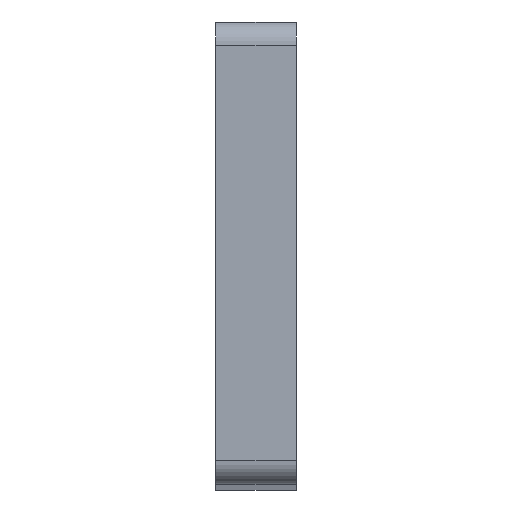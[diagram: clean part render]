
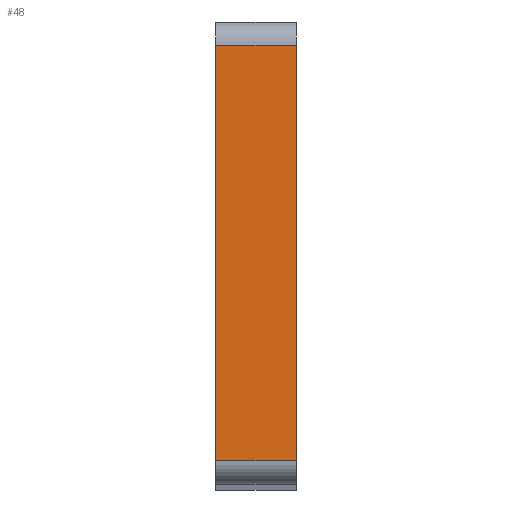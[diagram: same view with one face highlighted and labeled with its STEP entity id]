
A CAD part, top view. The second image highlights one B-rep face of the part: STEP entity #48.
In plain terms, the highlighted planar face has unit normal (0, 0, 1).
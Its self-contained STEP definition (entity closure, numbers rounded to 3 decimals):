
#1 = VERTEX_POINT ( 'NONE', #144 ) ;
#2 = VERTEX_POINT ( 'NONE', #148 ) ;
#8 = VERTEX_POINT ( 'NONE', #146 ) ;
#9 = VERTEX_POINT ( 'NONE', #147 ) ;
#19 = ORIENTED_EDGE ( 'NONE', *, *, #415, .T. ) ;
#26 = ORIENTED_EDGE ( 'NONE', *, *, #418, .T. ) ;
#28 = EDGE_LOOP ( 'NONE', ( #341, #26, #19, #34 ) ) ;
#34 = ORIENTED_EDGE ( 'NONE', *, *, #409, .T. ) ;
#48 = ADVANCED_FACE ( 'NONE', ( #291 ), #127, .F. ) ;
#124 = DIRECTION ( 'NONE',  ( -1., 0., 0. ) ) ;
#125 = DIRECTION ( 'NONE',  ( 0., 0., -1. ) ) ;
#127 = PLANE ( 'NONE',  #198 ) ;
#135 = CARTESIAN_POINT ( 'NONE',  ( 0.7, 0., 34. ) ) ;
#144 = CARTESIAN_POINT ( 'NONE',  ( 0., 3.8, 34. ) ) ;
#146 = CARTESIAN_POINT ( 'NONE',  ( 0.7, 3.8, 34. ) ) ;
#147 = CARTESIAN_POINT ( 'NONE',  ( 0.7, 0.2, 34. ) ) ;
#148 = CARTESIAN_POINT ( 'NONE',  ( 0., 0.2, 34. ) ) ;
#198 = AXIS2_PLACEMENT_3D ( 'NONE', #135, #125, #124 ) ;
#223 = VECTOR ( 'NONE', #477, 1000. ) ;
#228 = VECTOR ( 'NONE', #482, 1000. ) ;
#231 = LINE ( 'NONE', #483, #228 ) ;
#236 = LINE ( 'NONE', #493, #223 ) ;
#242 = VECTOR ( 'NONE', #495, 1000. ) ;
#244 = VECTOR ( 'NONE', #498, 1000. ) ;
#245 = LINE ( 'NONE', #497, #242 ) ;
#247 = LINE ( 'NONE', #499, #244 ) ;
#291 = FACE_OUTER_BOUND ( 'NONE', #28, .T. ) ;
#341 = ORIENTED_EDGE ( 'NONE', *, *, #408, .F. ) ;
#408 = EDGE_CURVE ( 'NONE', #8, #9, #247, .T. ) ;
#409 = EDGE_CURVE ( 'NONE', #2, #9, #245, .T. ) ;
#415 = EDGE_CURVE ( 'NONE', #1, #2, #231, .T. ) ;
#418 = EDGE_CURVE ( 'NONE', #8, #1, #236, .T. ) ;
#477 = DIRECTION ( 'NONE',  ( -1., 0., 0. ) ) ;
#482 = DIRECTION ( 'NONE',  ( 0., -1., 0. ) ) ;
#483 = CARTESIAN_POINT ( 'NONE',  ( 0., 0., 34. ) ) ;
#493 = CARTESIAN_POINT ( 'NONE',  ( 0.7, 3.8, 34. ) ) ;
#495 = DIRECTION ( 'NONE',  ( 1., 0., 0. ) ) ;
#497 = CARTESIAN_POINT ( 'NONE',  ( 0.7, 0.2, 34. ) ) ;
#498 = DIRECTION ( 'NONE',  ( 0., -1., 0. ) ) ;
#499 = CARTESIAN_POINT ( 'NONE',  ( 0.7, 0., 34. ) ) ;
